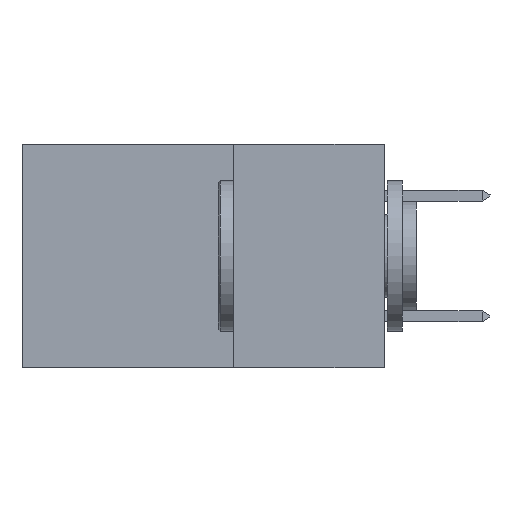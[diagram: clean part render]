
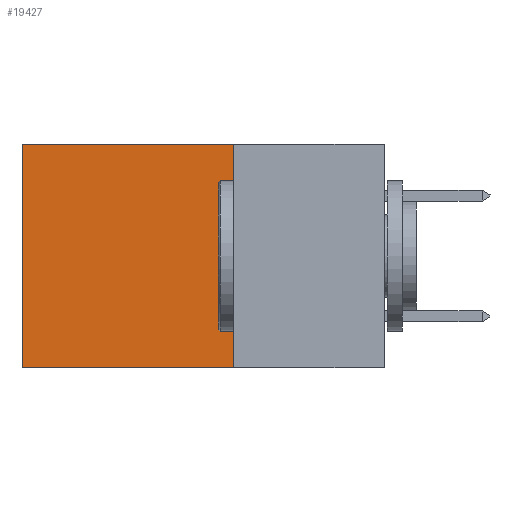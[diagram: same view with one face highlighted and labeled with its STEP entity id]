
A CAD part, left-side view. The second image highlights one B-rep face of the part: STEP entity #19427.
In plain terms, the highlighted planar face has unit normal (-1, 0, 0).
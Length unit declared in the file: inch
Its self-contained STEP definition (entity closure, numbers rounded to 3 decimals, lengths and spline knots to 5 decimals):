
#1270 = CARTESIAN_POINT ( 'NONE',  ( 0.2875, 0.25, -0.37 ) ) ;
#1453 = VERTEX_POINT ( 'NONE', #29114 ) ;
#3175 = ORIENTED_EDGE ( 'NONE', *, *, #32522, .T. ) ;
#4378 = EDGE_CURVE ( 'NONE', #25472, #26757, #27063, .T. ) ;
#4732 = DIRECTION ( 'NONE',  ( 1., 0., 0. ) ) ;
#4848 = PLANE ( 'NONE',  #34635 ) ;
#5103 = VECTOR ( 'NONE', #5835, 39.37008 ) ;
#5835 = DIRECTION ( 'NONE',  ( 0., 1., 0. ) ) ;
#6394 = CARTESIAN_POINT ( 'NONE',  ( 0.2875, 0.25, -0.37 ) ) ;
#6541 = DIRECTION ( 'NONE',  ( 0., 1., 0. ) ) ;
#10095 = EDGE_CURVE ( 'NONE', #29806, #25472, #25813, .T. ) ;
#12863 = CARTESIAN_POINT ( 'NONE',  ( 0.2875, 0.25, 0. ) ) ;
#13058 = EDGE_CURVE ( 'NONE', #1453, #26757, #22265, .T. ) ;
#13064 = ORIENTED_EDGE ( 'NONE', *, *, #10095, .F. ) ;
#13286 = CARTESIAN_POINT ( 'NONE',  ( 0.2875, 0.25, 0. ) ) ;
#13589 = DIRECTION ( 'NONE',  ( 0., 0., -1. ) ) ;
#15051 = LINE ( 'NONE', #20016, #29260 ) ;
#18785 = CARTESIAN_POINT ( 'NONE',  ( 0.2875, 0.6, 0. ) ) ;
#19173 = ORIENTED_EDGE ( 'NONE', *, *, #4378, .F. ) ;
#19427 = ADVANCED_FACE ( 'NONE', ( #32943 ), #4848, .F. ) ;
#20016 = CARTESIAN_POINT ( 'NONE',  ( 0.2875, 0.25, 0. ) ) ;
#21074 = VECTOR ( 'NONE', #22829, 39.37008 ) ;
#22265 = LINE ( 'NONE', #18785, #26161 ) ;
#22743 = EDGE_LOOP ( 'NONE', ( #27663, #19173, #13064, #3175 ) ) ;
#22829 = DIRECTION ( 'NONE',  ( 0., 0., -1. ) ) ;
#25472 = VERTEX_POINT ( 'NONE', #6394 ) ;
#25612 = CARTESIAN_POINT ( 'NONE',  ( 0.2875, 0.25, 0. ) ) ;
#25813 = LINE ( 'NONE', #25612, #21074 ) ;
#26161 = VECTOR ( 'NONE', #13589, 39.37008 ) ;
#26757 = VERTEX_POINT ( 'NONE', #28054 ) ;
#26982 = DIRECTION ( 'NONE',  ( 0., 0., -1. ) ) ;
#27063 = LINE ( 'NONE', #1270, #5103 ) ;
#27663 = ORIENTED_EDGE ( 'NONE', *, *, #13058, .T. ) ;
#28054 = CARTESIAN_POINT ( 'NONE',  ( 0.2875, 0.6, -0.37 ) ) ;
#29114 = CARTESIAN_POINT ( 'NONE',  ( 0.2875, 0.6, 0. ) ) ;
#29260 = VECTOR ( 'NONE', #6541, 39.37008 ) ;
#29806 = VERTEX_POINT ( 'NONE', #12863 ) ;
#32522 = EDGE_CURVE ( 'NONE', #29806, #1453, #15051, .T. ) ;
#32943 = FACE_OUTER_BOUND ( 'NONE', #22743, .T. ) ;
#34635 = AXIS2_PLACEMENT_3D ( 'NONE', #13286, #4732, #26982 ) ;
